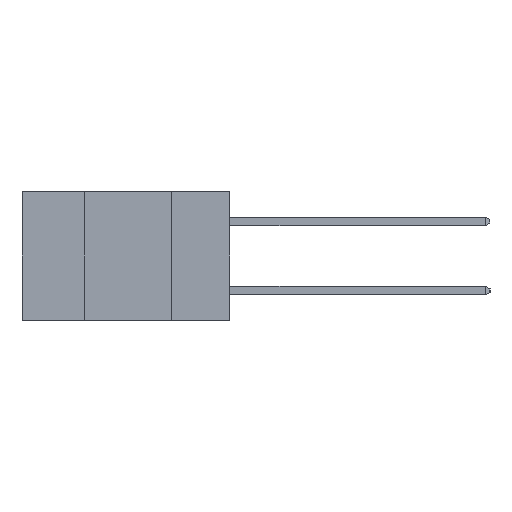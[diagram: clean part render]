
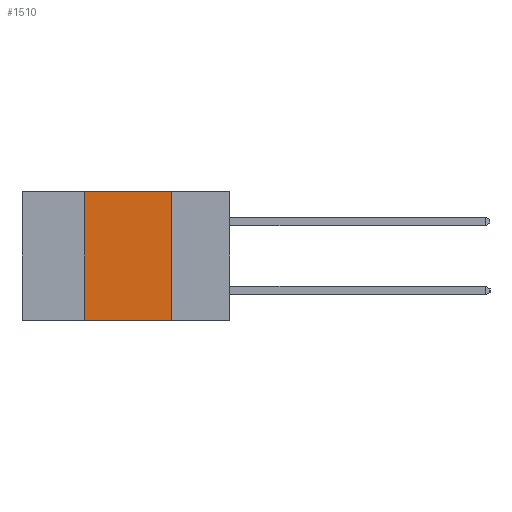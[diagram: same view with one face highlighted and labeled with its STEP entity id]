
A CAD part, left-side view. The second image highlights one B-rep face of the part: STEP entity #1510.
In plain terms, the highlighted planar face has unit normal (-1, 0, 0).
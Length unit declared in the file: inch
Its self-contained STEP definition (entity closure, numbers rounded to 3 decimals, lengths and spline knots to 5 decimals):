
#774 = CARTESIAN_POINT ( 'NONE',  ( 0., 0.17, -0.37 ) ) ;
#899 = CARTESIAN_POINT ( 'NONE',  ( 0., 0.6, 0. ) ) ;
#1217 = DIRECTION ( 'NONE',  ( 0., -1., 0. ) ) ;
#1510 = ADVANCED_FACE ( 'NONE', ( #10641 ), #24943, .F. ) ;
#4291 = AXIS2_PLACEMENT_3D ( 'NONE', #899, #23129, #22849 ) ;
#6739 = VECTOR ( 'NONE', #1217, 39.37008 ) ;
#6745 = DIRECTION ( 'NONE',  ( 0., -1., 0. ) ) ;
#7344 = VERTEX_POINT ( 'NONE', #774 ) ;
#7437 = ORIENTED_EDGE ( 'NONE', *, *, #8290, .F. ) ;
#7701 = LINE ( 'NONE', #10776, #22015 ) ;
#8290 = EDGE_CURVE ( 'NONE', #11729, #10183, #16164, .T. ) ;
#8462 = LINE ( 'NONE', #23015, #23359 ) ;
#10183 = VERTEX_POINT ( 'NONE', #20883 ) ;
#10641 = FACE_OUTER_BOUND ( 'NONE', #14859, .T. ) ;
#10776 = CARTESIAN_POINT ( 'NONE',  ( 0., 0.6, 0. ) ) ;
#11729 = VERTEX_POINT ( 'NONE', #23807 ) ;
#13195 = DIRECTION ( 'NONE',  ( 0., 0., 1. ) ) ;
#13226 = CARTESIAN_POINT ( 'NONE',  ( 0., 0.6, -0.37 ) ) ;
#13260 = ORIENTED_EDGE ( 'NONE', *, *, #20011, .F. ) ;
#13343 = DIRECTION ( 'NONE',  ( 0., 0., -1. ) ) ;
#13552 = VERTEX_POINT ( 'NONE', #23867 ) ;
#14859 = EDGE_LOOP ( 'NONE', ( #13260, #22968, #7437, #17224 ) ) ;
#15537 = VECTOR ( 'NONE', #13195, 39.37008 ) ;
#16164 = LINE ( 'NONE', #19033, #15537 ) ;
#17150 = LINE ( 'NONE', #13226, #6739 ) ;
#17224 = ORIENTED_EDGE ( 'NONE', *, *, #17446, .T. ) ;
#17446 = EDGE_CURVE ( 'NONE', #11729, #7344, #17150, .T. ) ;
#19033 = CARTESIAN_POINT ( 'NONE',  ( 0., 0.42, -0.37 ) ) ;
#20011 = EDGE_CURVE ( 'NONE', #13552, #7344, #8462, .T. ) ;
#20883 = CARTESIAN_POINT ( 'NONE',  ( 0., 0.42, 0. ) ) ;
#22015 = VECTOR ( 'NONE', #6745, 39.37008 ) ;
#22849 = DIRECTION ( 'NONE',  ( 0., 0., -1. ) ) ;
#22968 = ORIENTED_EDGE ( 'NONE', *, *, #23432, .F. ) ;
#23015 = CARTESIAN_POINT ( 'NONE',  ( 0., 0.17, -0.37 ) ) ;
#23129 = DIRECTION ( 'NONE',  ( 1., 0., 0. ) ) ;
#23359 = VECTOR ( 'NONE', #13343, 39.37008 ) ;
#23432 = EDGE_CURVE ( 'NONE', #10183, #13552, #7701, .T. ) ;
#23807 = CARTESIAN_POINT ( 'NONE',  ( 0., 0.42, -0.37 ) ) ;
#23867 = CARTESIAN_POINT ( 'NONE',  ( 0., 0.17, 0. ) ) ;
#24943 = PLANE ( 'NONE',  #4291 ) ;
